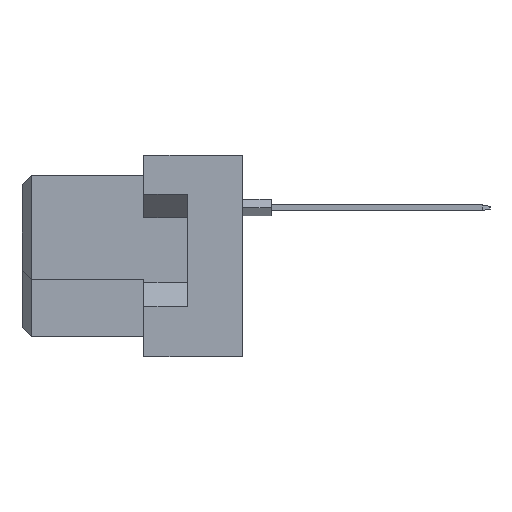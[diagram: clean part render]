
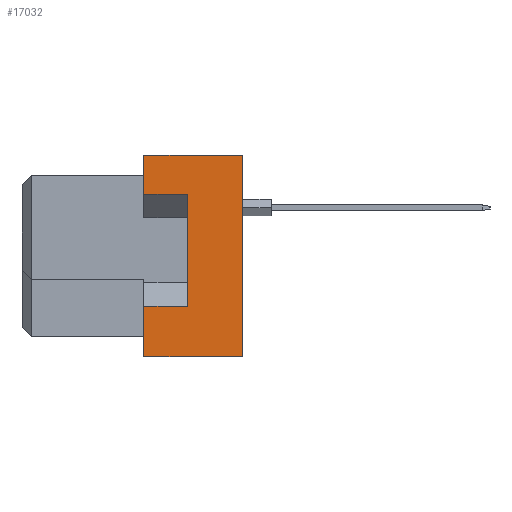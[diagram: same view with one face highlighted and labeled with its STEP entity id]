
A CAD part, left-side view. The second image highlights one B-rep face of the part: STEP entity #17032.
In plain terms, the highlighted planar face has unit normal (-1, 0, 0).
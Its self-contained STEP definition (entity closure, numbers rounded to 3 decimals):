
#79 = ORIENTED_EDGE ( 'NONE', *, *, #23464, .F. ) ;
#295 = FACE_OUTER_BOUND ( 'NONE', #14851, .T. ) ;
#480 = DIRECTION ( 'NONE',  ( -1., 0., 0. ) ) ;
#932 = DIRECTION ( 'NONE',  ( 0., 0., 1. ) ) ;
#1790 = VERTEX_POINT ( 'NONE', #30274 ) ;
#2390 = ORIENTED_EDGE ( 'NONE', *, *, #12208, .F. ) ;
#2544 = CARTESIAN_POINT ( 'NONE',  ( -47.5, -8.7, -2.65 ) ) ;
#2914 = EDGE_CURVE ( 'NONE', #14152, #24217, #23679, .T. ) ;
#3260 = CARTESIAN_POINT ( 'NONE',  ( -47.5, -6.4, -5.3 ) ) ;
#3462 = LINE ( 'NONE', #3260, #21837 ) ;
#3964 = AXIS2_PLACEMENT_3D ( 'NONE', #36019, #480, #17972 ) ;
#4152 = CARTESIAN_POINT ( 'NONE',  ( -47.5, -8.7, 3.25 ) ) ;
#4342 = CARTESIAN_POINT ( 'NONE',  ( -47.5, -6.4, -5.3 ) ) ;
#4406 = DIRECTION ( 'NONE',  ( 0., 0., 1. ) ) ;
#5029 = VERTEX_POINT ( 'NONE', #11402 ) ;
#5655 = CARTESIAN_POINT ( 'NONE',  ( -47.5, -11.6, 5.3 ) ) ;
#6057 = ORIENTED_EDGE ( 'NONE', *, *, #2914, .T. ) ;
#6180 = CARTESIAN_POINT ( 'NONE',  ( -47.5, -11.6, 5.3 ) ) ;
#6494 = EDGE_CURVE ( 'NONE', #1790, #14152, #28856, .T. ) ;
#7725 = LINE ( 'NONE', #22297, #16563 ) ;
#7870 = DIRECTION ( 'NONE',  ( 0., 0., 1. ) ) ;
#8282 = EDGE_CURVE ( 'NONE', #1790, #5029, #20450, .T. ) ;
#8341 = VECTOR ( 'NONE', #29704, 1000. ) ;
#10755 = VECTOR ( 'NONE', #38200, 1000. ) ;
#11402 = CARTESIAN_POINT ( 'NONE',  ( -47.5, -6.4, -5.3 ) ) ;
#11894 = VERTEX_POINT ( 'NONE', #26364 ) ;
#11987 = EDGE_CURVE ( 'NONE', #31940, #34694, #37810, .T. ) ;
#12208 = EDGE_CURVE ( 'NONE', #5029, #34694, #13098, .T. ) ;
#12416 = DIRECTION ( 'NONE',  ( 0., 1., 0. ) ) ;
#12522 = PLANE ( 'NONE',  #3964 ) ;
#13083 = CARTESIAN_POINT ( 'NONE',  ( -47.5, -6.4, -2.65 ) ) ;
#13098 = LINE ( 'NONE', #4342, #36171 ) ;
#13164 = ORIENTED_EDGE ( 'NONE', *, *, #6494, .T. ) ;
#14152 = VERTEX_POINT ( 'NONE', #5655 ) ;
#14851 = EDGE_LOOP ( 'NONE', ( #36254, #2390, #30947, #13164, #6057, #33470, #79, #29839 ) ) ;
#16276 = VERTEX_POINT ( 'NONE', #4152 ) ;
#16563 = VECTOR ( 'NONE', #4406, 1000. ) ;
#16831 = VECTOR ( 'NONE', #12416, 1000. ) ;
#17032 = ADVANCED_FACE ( 'NONE', ( #295 ), #12522, .T. ) ;
#17349 = CARTESIAN_POINT ( 'NONE',  ( -47.5, -11.6, -5.3 ) ) ;
#17415 = CARTESIAN_POINT ( 'NONE',  ( -47.5, -8.7, -2.65 ) ) ;
#17972 = DIRECTION ( 'NONE',  ( 0., 0., 1. ) ) ;
#20450 = LINE ( 'NONE', #17349, #33527 ) ;
#20773 = EDGE_CURVE ( 'NONE', #31940, #16276, #7725, .T. ) ;
#21837 = VECTOR ( 'NONE', #932, 1000. ) ;
#21850 = DIRECTION ( 'NONE',  ( 0., 0., 1. ) ) ;
#22281 = VECTOR ( 'NONE', #7870, 1000. ) ;
#22297 = CARTESIAN_POINT ( 'NONE',  ( -47.5, -8.7, -2.65 ) ) ;
#23464 = EDGE_CURVE ( 'NONE', #16276, #11894, #35545, .T. ) ;
#23679 = LINE ( 'NONE', #6180, #8341 ) ;
#24127 = CARTESIAN_POINT ( 'NONE',  ( -47.5, -6.4, 5.3 ) ) ;
#24217 = VERTEX_POINT ( 'NONE', #24127 ) ;
#26364 = CARTESIAN_POINT ( 'NONE',  ( -47.5, -6.4, 3.25 ) ) ;
#28856 = LINE ( 'NONE', #37198, #22281 ) ;
#29704 = DIRECTION ( 'NONE',  ( 0., 1., 0. ) ) ;
#29839 = ORIENTED_EDGE ( 'NONE', *, *, #20773, .F. ) ;
#30274 = CARTESIAN_POINT ( 'NONE',  ( -47.5, -11.6, -5.3 ) ) ;
#30342 = EDGE_CURVE ( 'NONE', #11894, #24217, #3462, .T. ) ;
#30947 = ORIENTED_EDGE ( 'NONE', *, *, #8282, .F. ) ;
#31940 = VERTEX_POINT ( 'NONE', #2544 ) ;
#33470 = ORIENTED_EDGE ( 'NONE', *, *, #30342, .F. ) ;
#33527 = VECTOR ( 'NONE', #38322, 1000. ) ;
#34694 = VERTEX_POINT ( 'NONE', #13083 ) ;
#35545 = LINE ( 'NONE', #35919, #16831 ) ;
#35919 = CARTESIAN_POINT ( 'NONE',  ( -47.5, -8.7, 3.25 ) ) ;
#36019 = CARTESIAN_POINT ( 'NONE',  ( -47.5, -11.6, 5.3 ) ) ;
#36171 = VECTOR ( 'NONE', #21850, 1000. ) ;
#36254 = ORIENTED_EDGE ( 'NONE', *, *, #11987, .T. ) ;
#37198 = CARTESIAN_POINT ( 'NONE',  ( -47.5, -11.6, 5.3 ) ) ;
#37810 = LINE ( 'NONE', #17415, #10755 ) ;
#38200 = DIRECTION ( 'NONE',  ( 0., 1., 0. ) ) ;
#38322 = DIRECTION ( 'NONE',  ( 0., 1., 0. ) ) ;
